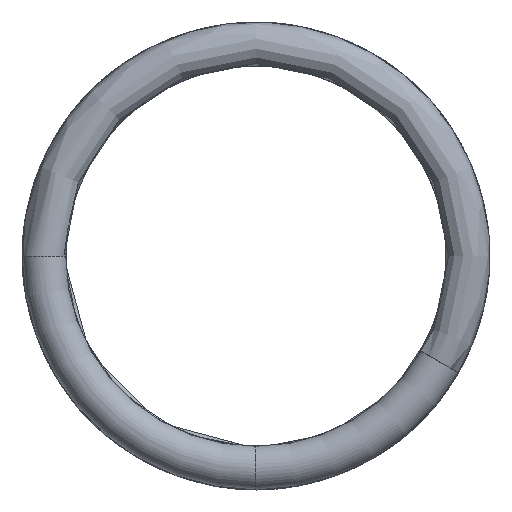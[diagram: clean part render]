
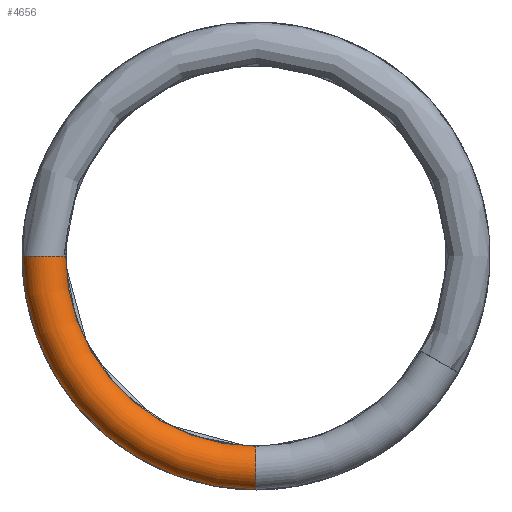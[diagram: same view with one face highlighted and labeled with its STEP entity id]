
A CAD part, front view. The second image highlights one B-rep face of the part: STEP entity #4656.
In plain terms, the highlighted toroidal (fillet/blend) face has major radius 5.182 mm and minor radius 0.533 mm.
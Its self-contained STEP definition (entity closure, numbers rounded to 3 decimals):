
#1 = CARTESIAN_POINT ( 'NONE',  ( -4.648, 0.533, 0. ) ) ;
#19 = CARTESIAN_POINT ( 'NONE',  ( -5.715, 0.394, 0. ) ) ;
#413 = DIRECTION ( 'NONE',  ( -1., 0., 0. ) ) ;
#434 = CIRCLE ( 'NONE', #4778, 4.648 ) ;
#489 = CARTESIAN_POINT ( 'NONE',  ( -5.715, 0.533, 0. ) ) ;
#730 = VERTEX_POINT ( 'NONE', #489 ) ;
#1417 = VERTEX_POINT ( 'NONE', #1710 ) ;
#1457 = B_SPLINE_CURVE_WITH_KNOTS ( 'NONE', 3,
 ( #4364, #3387, #4868, #1952, #5354, #2438, #5845, #2918, #19, #3406 ),
 .UNSPECIFIED., .F., .F.,
 ( 4, 2, 2, 2, 4 ),
 ( 0., 0.25, 0.5, 0.75, 1. ),
 .UNSPECIFIED. ) ;
#1487 = CARTESIAN_POINT ( 'NONE',  ( 0., 0.533, 0. ) ) ;
#1557 = EDGE_LOOP ( 'NONE', ( #1719, #3147, #2986, #2851 ) ) ;
#1674 = DIRECTION ( 'NONE',  ( 0., -1., 0. ) ) ;
#1710 = CARTESIAN_POINT ( 'NONE',  ( 0., 0.533, -5.715 ) ) ;
#1719 = ORIENTED_EDGE ( 'NONE', *, *, #5677, .T. ) ;
#1882 = TOROIDAL_SURFACE ( 'NONE', #4860, 5.182, 0.533 ) ;
#1952 = CARTESIAN_POINT ( 'NONE',  ( -4.903, 0.057, 0. ) ) ;
#1971 = DIRECTION ( 'NONE',  ( 0., 0., -1. ) ) ;
#2160 = CARTESIAN_POINT ( 'NONE',  ( 0., 0.533, 0. ) ) ;
#2192 = CARTESIAN_POINT ( 'NONE',  ( 0., 0.533, -4.648 ) ) ;
#2438 = CARTESIAN_POINT ( 'NONE',  ( -5.321, 0., 0. ) ) ;
#2725 = CARTESIAN_POINT ( 'NONE',  ( 0., 0.533, 0. ) ) ;
#2851 = ORIENTED_EDGE ( 'NONE', *, *, #5156, .F. ) ;
#2918 = CARTESIAN_POINT ( 'NONE',  ( -5.658, 0.255, 0. ) ) ;
#2986 = ORIENTED_EDGE ( 'NONE', *, *, #5388, .T. ) ;
#3147 = ORIENTED_EDGE ( 'NONE', *, *, #5715, .T. ) ;
#3208 = DIRECTION ( 'NONE',  ( 0., 0., -1. ) ) ;
#3312 = CARTESIAN_POINT ( 'NONE',  ( 0., 0.533, -5.182 ) ) ;
#3387 = CARTESIAN_POINT ( 'NONE',  ( -4.648, 0.394, 0. ) ) ;
#3400 = DIRECTION ( 'NONE',  ( 0., 0., -1. ) ) ;
#3406 = CARTESIAN_POINT ( 'NONE',  ( -5.715, 0.533, 0. ) ) ;
#3796 = DIRECTION ( 'NONE',  ( 0., 0., 1. ) ) ;
#3972 = VERTEX_POINT ( 'NONE', #2192 ) ;
#4207 = AXIS2_PLACEMENT_3D ( 'NONE', #1487, #4887, #1971 ) ;
#4314 = AXIS2_PLACEMENT_3D ( 'NONE', #3312, #413, #3796 ) ;
#4364 = CARTESIAN_POINT ( 'NONE',  ( -4.648, 0.533, 0. ) ) ;
#4656 = ADVANCED_FACE ( 'NONE', ( #5303 ), #1882, .T. ) ;
#4778 = AXIS2_PLACEMENT_3D ( 'NONE', #2725, #6130, #3208 ) ;
#4860 = AXIS2_PLACEMENT_3D ( 'NONE', #2160, #1674, #3400 ) ;
#4868 = CARTESIAN_POINT ( 'NONE',  ( -4.706, 0.255, 0. ) ) ;
#4887 = DIRECTION ( 'NONE',  ( 0., -1., 0. ) ) ;
#4906 = CIRCLE ( 'NONE', #4207, 5.715 ) ;
#5064 = CIRCLE ( 'NONE', #4314, 0.533 ) ;
#5156 = EDGE_CURVE ( 'NONE', #5675, #3972, #434, .T. ) ;
#5303 = FACE_OUTER_BOUND ( 'NONE', #1557, .T. ) ;
#5354 = CARTESIAN_POINT ( 'NONE',  ( -5.042, 0., 0. ) ) ;
#5388 = EDGE_CURVE ( 'NONE', #1417, #3972, #5064, .T. ) ;
#5675 = VERTEX_POINT ( 'NONE', #1 ) ;
#5677 = EDGE_CURVE ( 'NONE', #5675, #730, #1457, .T. ) ;
#5715 = EDGE_CURVE ( 'NONE', #730, #1417, #4906, .T. ) ;
#5845 = CARTESIAN_POINT ( 'NONE',  ( -5.46, 0.057, 0. ) ) ;
#6130 = DIRECTION ( 'NONE',  ( 0., -1., 0. ) ) ;
